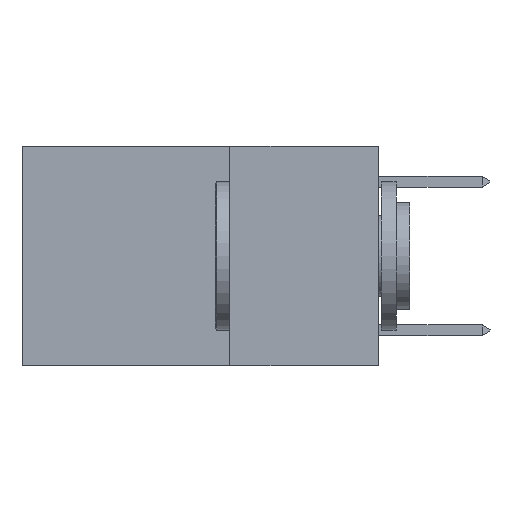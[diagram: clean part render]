
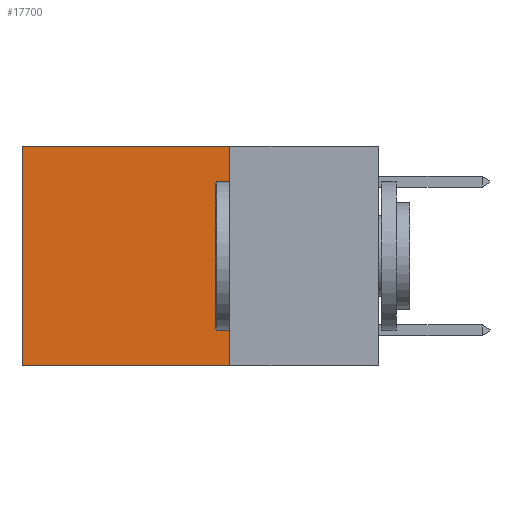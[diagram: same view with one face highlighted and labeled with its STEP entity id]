
A CAD part, left-side view. The second image highlights one B-rep face of the part: STEP entity #17700.
In plain terms, the highlighted planar face has unit normal (-1, 0, 0).
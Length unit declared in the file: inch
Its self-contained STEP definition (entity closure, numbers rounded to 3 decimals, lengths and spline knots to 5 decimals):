
#333 = ORIENTED_EDGE ( 'NONE', *, *, #12621, .F. ) ;
#769 = VERTEX_POINT ( 'NONE', #13331 ) ;
#802 = VERTEX_POINT ( 'NONE', #19056 ) ;
#1307 = ORIENTED_EDGE ( 'NONE', *, *, #16360, .T. ) ;
#1518 = ORIENTED_EDGE ( 'NONE', *, *, #3838, .T. ) ;
#2623 = VERTEX_POINT ( 'NONE', #24048 ) ;
#3495 = LINE ( 'NONE', #20901, #13063 ) ;
#3838 = EDGE_CURVE ( 'NONE', #5152, #802, #15629, .T. ) ;
#5063 = DIRECTION ( 'NONE',  ( 0., 1., 0. ) ) ;
#5152 = VERTEX_POINT ( 'NONE', #15175 ) ;
#5579 = VECTOR ( 'NONE', #13589, 39.37008 ) ;
#6322 = CARTESIAN_POINT ( 'NONE',  ( 0.2625, 0.25, 0. ) ) ;
#7913 = CARTESIAN_POINT ( 'NONE',  ( 0.2625, 0.6, 0. ) ) ;
#8223 = DIRECTION ( 'NONE',  ( 1., 0., 0. ) ) ;
#12621 = EDGE_CURVE ( 'NONE', #2623, #802, #20835, .T. ) ;
#12885 = ORIENTED_EDGE ( 'NONE', *, *, #18238, .F. ) ;
#13063 = VECTOR ( 'NONE', #17246, 39.37008 ) ;
#13331 = CARTESIAN_POINT ( 'NONE',  ( 0.2625, 0.25, 0. ) ) ;
#13371 = LINE ( 'NONE', #19109, #17766 ) ;
#13589 = DIRECTION ( 'NONE',  ( 0., 0., -1. ) ) ;
#14183 = FACE_OUTER_BOUND ( 'NONE', #23666, .T. ) ;
#14513 = CARTESIAN_POINT ( 'NONE',  ( 0.2625, 0.25, -0.37 ) ) ;
#15175 = CARTESIAN_POINT ( 'NONE',  ( 0.2625, 0.6, 0. ) ) ;
#15287 = VECTOR ( 'NONE', #5063, 39.37008 ) ;
#15629 = LINE ( 'NONE', #7913, #5579 ) ;
#16360 = EDGE_CURVE ( 'NONE', #769, #5152, #3495, .T. ) ;
#17246 = DIRECTION ( 'NONE',  ( 0., 1., 0. ) ) ;
#17588 = PLANE ( 'NONE',  #24182 ) ;
#17700 = ADVANCED_FACE ( 'NONE', ( #14183 ), #17588, .F. ) ;
#17766 = VECTOR ( 'NONE', #22775, 39.37008 ) ;
#18238 = EDGE_CURVE ( 'NONE', #769, #2623, #13371, .T. ) ;
#19056 = CARTESIAN_POINT ( 'NONE',  ( 0.2625, 0.6, -0.37 ) ) ;
#19109 = CARTESIAN_POINT ( 'NONE',  ( 0.2625, 0.25, 0. ) ) ;
#20835 = LINE ( 'NONE', #14513, #15287 ) ;
#20901 = CARTESIAN_POINT ( 'NONE',  ( 0.2625, 0.25, 0. ) ) ;
#21327 = DIRECTION ( 'NONE',  ( 0., 0., -1. ) ) ;
#22775 = DIRECTION ( 'NONE',  ( 0., 0., -1. ) ) ;
#23666 = EDGE_LOOP ( 'NONE', ( #1518, #333, #12885, #1307 ) ) ;
#24048 = CARTESIAN_POINT ( 'NONE',  ( 0.2625, 0.25, -0.37 ) ) ;
#24182 = AXIS2_PLACEMENT_3D ( 'NONE', #6322, #8223, #21327 ) ;
